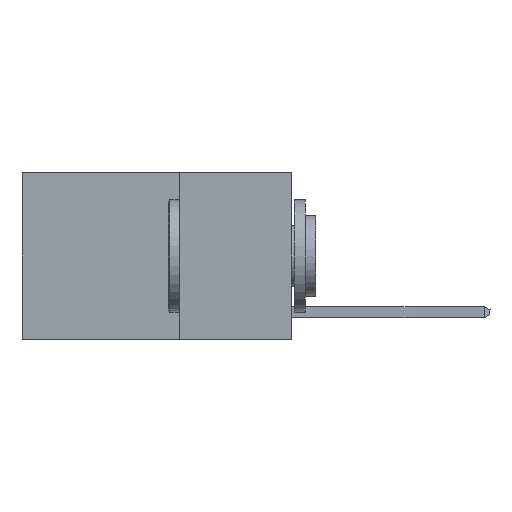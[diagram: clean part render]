
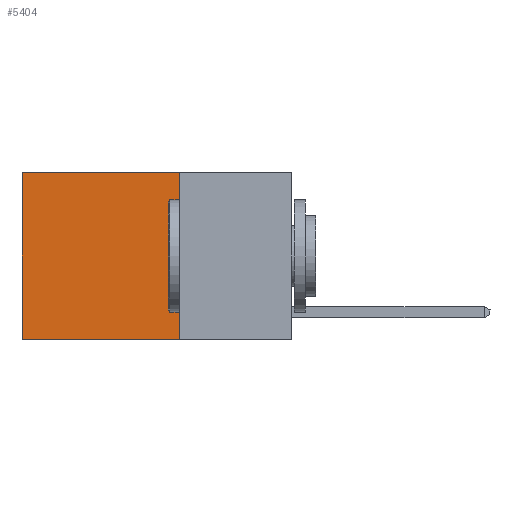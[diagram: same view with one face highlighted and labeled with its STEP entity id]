
A CAD part, left-side view. The second image highlights one B-rep face of the part: STEP entity #5404.
In plain terms, the highlighted planar face has unit normal (-1, 0, 0).
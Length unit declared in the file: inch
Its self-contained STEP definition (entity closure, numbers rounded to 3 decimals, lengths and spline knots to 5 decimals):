
#1159 = LINE ( 'NONE', #11619, #10737 ) ;
#1569 = DIRECTION ( 'NONE',  ( 0., 0., -1. ) ) ;
#1780 = DIRECTION ( 'NONE',  ( 0., 0., -1. ) ) ;
#1837 = CARTESIAN_POINT ( 'NONE',  ( 0.2625, 0.6, 0. ) ) ;
#1879 = CARTESIAN_POINT ( 'NONE',  ( 0.2625, 0.25, 0. ) ) ;
#2520 = EDGE_LOOP ( 'NONE', ( #7853, #15440, #9504, #5542 ) ) ;
#2706 = VERTEX_POINT ( 'NONE', #8345 ) ;
#3327 = EDGE_CURVE ( 'NONE', #14060, #14362, #8206, .T. ) ;
#3862 = LINE ( 'NONE', #9064, #10075 ) ;
#4247 = DIRECTION ( 'NONE',  ( 1., 0., 0. ) ) ;
#5305 = VECTOR ( 'NONE', #1780, 39.37008 ) ;
#5404 = ADVANCED_FACE ( 'NONE', ( #9674 ), #10429, .F. ) ;
#5534 = DIRECTION ( 'NONE',  ( 0., 1., 0. ) ) ;
#5542 = ORIENTED_EDGE ( 'NONE', *, *, #8550, .T. ) ;
#7853 = ORIENTED_EDGE ( 'NONE', *, *, #3327, .T. ) ;
#8206 = LINE ( 'NONE', #1837, #5305 ) ;
#8345 = CARTESIAN_POINT ( 'NONE',  ( 0.2625, 0.25, -0.37 ) ) ;
#8423 = CARTESIAN_POINT ( 'NONE',  ( 0.2625, 0.6, -0.37 ) ) ;
#8550 = EDGE_CURVE ( 'NONE', #8639, #14060, #1159, .T. ) ;
#8639 = VERTEX_POINT ( 'NONE', #1879 ) ;
#9064 = CARTESIAN_POINT ( 'NONE',  ( 0.2625, 0.25, 0. ) ) ;
#9504 = ORIENTED_EDGE ( 'NONE', *, *, #10291, .F. ) ;
#9674 = FACE_OUTER_BOUND ( 'NONE', #2520, .T. ) ;
#10075 = VECTOR ( 'NONE', #1569, 39.37008 ) ;
#10291 = EDGE_CURVE ( 'NONE', #8639, #2706, #3862, .T. ) ;
#10429 = PLANE ( 'NONE',  #15802 ) ;
#10737 = VECTOR ( 'NONE', #5534, 39.37008 ) ;
#11383 = LINE ( 'NONE', #12574, #14273 ) ;
#11619 = CARTESIAN_POINT ( 'NONE',  ( 0.2625, 0.25, 0. ) ) ;
#12015 = EDGE_CURVE ( 'NONE', #2706, #14362, #11383, .T. ) ;
#12573 = CARTESIAN_POINT ( 'NONE',  ( 0.2625, 0.6, 0. ) ) ;
#12574 = CARTESIAN_POINT ( 'NONE',  ( 0.2625, 0.25, -0.37 ) ) ;
#12909 = DIRECTION ( 'NONE',  ( 0., 0., -1. ) ) ;
#13820 = DIRECTION ( 'NONE',  ( 0., 1., 0. ) ) ;
#14060 = VERTEX_POINT ( 'NONE', #12573 ) ;
#14273 = VECTOR ( 'NONE', #13820, 39.37008 ) ;
#14362 = VERTEX_POINT ( 'NONE', #8423 ) ;
#15295 = CARTESIAN_POINT ( 'NONE',  ( 0.2625, 0.25, 0. ) ) ;
#15440 = ORIENTED_EDGE ( 'NONE', *, *, #12015, .F. ) ;
#15802 = AXIS2_PLACEMENT_3D ( 'NONE', #15295, #4247, #12909 ) ;
